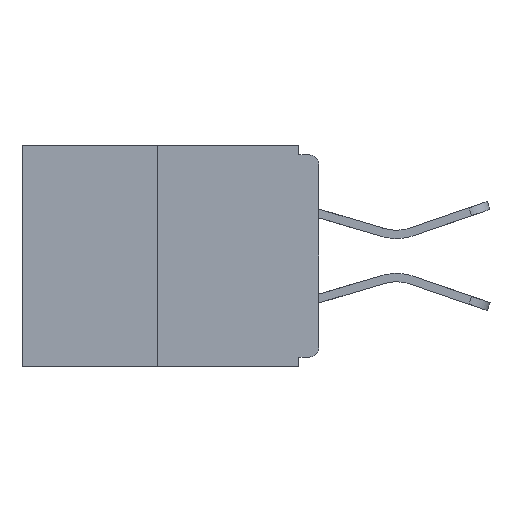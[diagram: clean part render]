
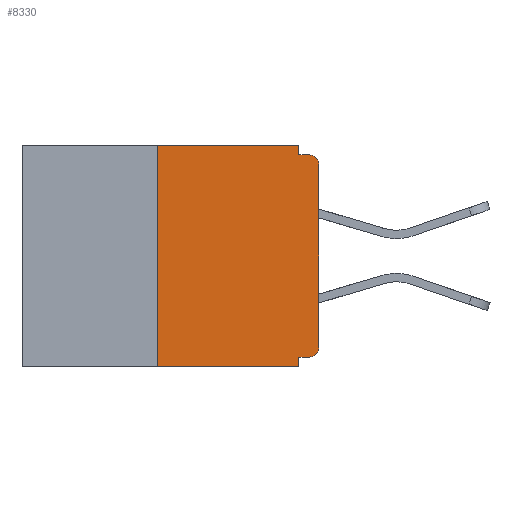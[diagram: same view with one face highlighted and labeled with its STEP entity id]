
A CAD part, left-side view. The second image highlights one B-rep face of the part: STEP entity #8330.
In plain terms, the highlighted planar face has unit normal (-1, 0, 0).
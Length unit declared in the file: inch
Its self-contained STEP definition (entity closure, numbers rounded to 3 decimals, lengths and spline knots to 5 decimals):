
#102 = DIRECTION ( 'NONE',  ( -1., 0., 0. ) ) ;
#1674 = EDGE_CURVE ( 'NONE', #3100, #10945, #15541, .T. ) ;
#1791 = CARTESIAN_POINT ( 'NONE',  ( 0., 0.031, -0.015 ) ) ;
#2331 = EDGE_CURVE ( 'NONE', #15414, #16652, #7574, .T. ) ;
#2353 = ORIENTED_EDGE ( 'NONE', *, *, #1674, .F. ) ;
#2412 = DIRECTION ( 'NONE',  ( 0., 0., -1. ) ) ;
#2680 = VECTOR ( 'NONE', #7805, 39.37008 ) ;
#3054 = CARTESIAN_POINT ( 'NONE',  ( 0., 0.031, 0. ) ) ;
#3100 = VERTEX_POINT ( 'NONE', #14039 ) ;
#3102 = VERTEX_POINT ( 'NONE', #10299 ) ;
#3107 = EDGE_CURVE ( 'NONE', #10945, #12190, #12807, .T. ) ;
#3250 = CIRCLE ( 'NONE', #14143, 0.015 ) ;
#3907 = DIRECTION ( 'NONE',  ( 0., 0., -1. ) ) ;
#3950 = CARTESIAN_POINT ( 'NONE',  ( 0., 0.031, -0.343 ) ) ;
#4247 = DIRECTION ( 'NONE',  ( 0., 0., -1. ) ) ;
#4309 = ORIENTED_EDGE ( 'NONE', *, *, #15886, .T. ) ;
#5389 = DIRECTION ( 'NONE',  ( 0., 0., -1. ) ) ;
#5663 = VECTOR ( 'NONE', #7759, 39.37008 ) ;
#5859 = AXIS2_PLACEMENT_3D ( 'NONE', #17092, #17145, #2412 ) ;
#5877 = CARTESIAN_POINT ( 'NONE',  ( 0., 0.25, -0.343 ) ) ;
#5953 = ORIENTED_EDGE ( 'NONE', *, *, #15589, .T. ) ;
#6049 = LINE ( 'NONE', #7142, #9639 ) ;
#6283 = CARTESIAN_POINT ( 'NONE',  ( 0., 0.015, -0.015 ) ) ;
#6431 = CARTESIAN_POINT ( 'NONE',  ( 0., 0.031, -0.328 ) ) ;
#6701 = VECTOR ( 'NONE', #9287, 39.37008 ) ;
#7142 = CARTESIAN_POINT ( 'NONE',  ( 0., 0., -0.015 ) ) ;
#7149 = EDGE_CURVE ( 'NONE', #9144, #3102, #7931, .T. ) ;
#7304 = CARTESIAN_POINT ( 'NONE',  ( 0., 0., 0. ) ) ;
#7452 = CARTESIAN_POINT ( 'NONE',  ( 0., 0.031, 0. ) ) ;
#7466 = CARTESIAN_POINT ( 'NONE',  ( 0., 0.031, -0.343 ) ) ;
#7574 = LINE ( 'NONE', #7452, #17180 ) ;
#7759 = DIRECTION ( 'NONE',  ( 0., 1., 0. ) ) ;
#7805 = DIRECTION ( 'NONE',  ( 0., 0., 1. ) ) ;
#7897 = EDGE_LOOP ( 'NONE', ( #8781, #9196, #5953, #16081, #2353, #14576, #15747, #4309, #16270, #17036 ) ) ;
#7901 = CARTESIAN_POINT ( 'NONE',  ( 0., 0.46, 0. ) ) ;
#7931 = LINE ( 'NONE', #13132, #2680 ) ;
#8014 = LINE ( 'NONE', #17285, #6701 ) ;
#8084 = CARTESIAN_POINT ( 'NONE',  ( 0., 0.015, -0.313 ) ) ;
#8168 = VERTEX_POINT ( 'NONE', #11934 ) ;
#8330 = ADVANCED_FACE ( 'NONE', ( #16261 ), #13224, .F. ) ;
#8781 = ORIENTED_EDGE ( 'NONE', *, *, #13296, .F. ) ;
#8955 = VECTOR ( 'NONE', #15275, 39.37008 ) ;
#9074 = VERTEX_POINT ( 'NONE', #6283 ) ;
#9144 = VERTEX_POINT ( 'NONE', #5877 ) ;
#9196 = ORIENTED_EDGE ( 'NONE', *, *, #7149, .F. ) ;
#9287 = DIRECTION ( 'NONE',  ( 0., -1., 0. ) ) ;
#9639 = VECTOR ( 'NONE', #16498, 39.37008 ) ;
#9688 = CARTESIAN_POINT ( 'NONE',  ( 0., 0., -0.03 ) ) ;
#10093 = CIRCLE ( 'NONE', #5859, 0.015 ) ;
#10190 = LINE ( 'NONE', #11063, #14555 ) ;
#10299 = CARTESIAN_POINT ( 'NONE',  ( 0., 0.25, 0. ) ) ;
#10945 = VERTEX_POINT ( 'NONE', #6431 ) ;
#11063 = CARTESIAN_POINT ( 'NONE',  ( 0., 0.46, 0. ) ) ;
#11100 = EDGE_CURVE ( 'NONE', #16652, #9074, #6049, .T. ) ;
#11142 = VECTOR ( 'NONE', #4247, 39.37008 ) ;
#11609 = DIRECTION ( 'NONE',  ( 0., 0., -1. ) ) ;
#11934 = CARTESIAN_POINT ( 'NONE',  ( 0., 0., -0.313 ) ) ;
#12021 = DIRECTION ( 'NONE',  ( 1., 0., 0. ) ) ;
#12190 = VERTEX_POINT ( 'NONE', #7466 ) ;
#12546 = EDGE_CURVE ( 'NONE', #8168, #16099, #13934, .T. ) ;
#12807 = LINE ( 'NONE', #3950, #11142 ) ;
#13132 = CARTESIAN_POINT ( 'NONE',  ( 0., 0.25, 0. ) ) ;
#13224 = PLANE ( 'NONE',  #15364 ) ;
#13296 = EDGE_CURVE ( 'NONE', #3102, #15414, #10190, .T. ) ;
#13879 = EDGE_CURVE ( 'NONE', #3100, #8168, #3250, .T. ) ;
#13934 = LINE ( 'NONE', #7304, #8955 ) ;
#14039 = CARTESIAN_POINT ( 'NONE',  ( 0., 0.015, -0.328 ) ) ;
#14143 = AXIS2_PLACEMENT_3D ( 'NONE', #8084, #102, #5389 ) ;
#14410 = CARTESIAN_POINT ( 'NONE',  ( 0., 0., -0.328 ) ) ;
#14555 = VECTOR ( 'NONE', #16276, 39.37008 ) ;
#14576 = ORIENTED_EDGE ( 'NONE', *, *, #13879, .T. ) ;
#15275 = DIRECTION ( 'NONE',  ( 0., 0., 1. ) ) ;
#15364 = AXIS2_PLACEMENT_3D ( 'NONE', #7901, #12021, #3907 ) ;
#15414 = VERTEX_POINT ( 'NONE', #3054 ) ;
#15541 = LINE ( 'NONE', #14410, #5663 ) ;
#15589 = EDGE_CURVE ( 'NONE', #9144, #12190, #8014, .T. ) ;
#15747 = ORIENTED_EDGE ( 'NONE', *, *, #12546, .T. ) ;
#15886 = EDGE_CURVE ( 'NONE', #16099, #9074, #10093, .T. ) ;
#16081 = ORIENTED_EDGE ( 'NONE', *, *, #3107, .F. ) ;
#16099 = VERTEX_POINT ( 'NONE', #9688 ) ;
#16261 = FACE_OUTER_BOUND ( 'NONE', #7897, .T. ) ;
#16270 = ORIENTED_EDGE ( 'NONE', *, *, #11100, .F. ) ;
#16276 = DIRECTION ( 'NONE',  ( 0., -1., 0. ) ) ;
#16498 = DIRECTION ( 'NONE',  ( 0., -1., 0. ) ) ;
#16652 = VERTEX_POINT ( 'NONE', #1791 ) ;
#17036 = ORIENTED_EDGE ( 'NONE', *, *, #2331, .F. ) ;
#17092 = CARTESIAN_POINT ( 'NONE',  ( 0., 0.015, -0.03 ) ) ;
#17145 = DIRECTION ( 'NONE',  ( -1., 0., 0. ) ) ;
#17180 = VECTOR ( 'NONE', #11609, 39.37008 ) ;
#17285 = CARTESIAN_POINT ( 'NONE',  ( 0., 0.46, -0.343 ) ) ;
